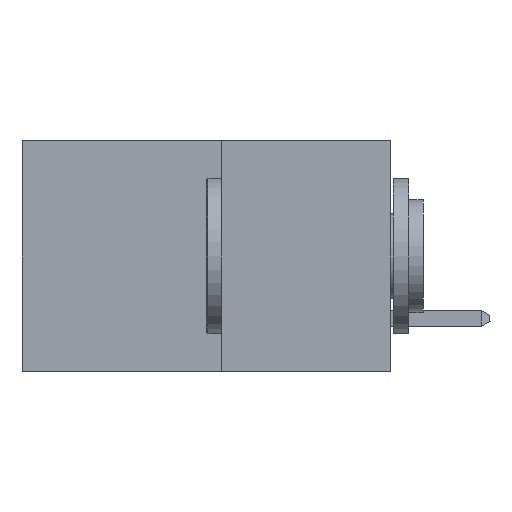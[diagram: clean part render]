
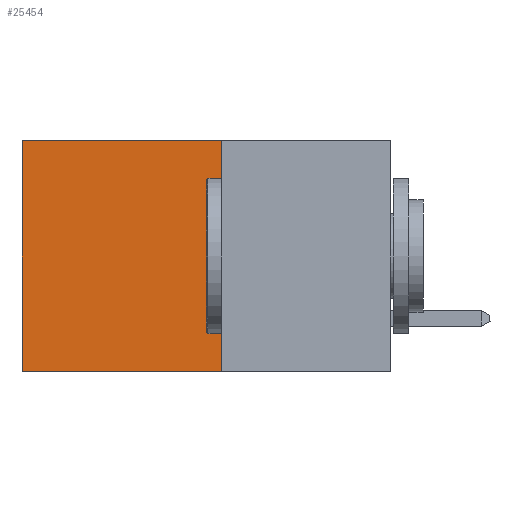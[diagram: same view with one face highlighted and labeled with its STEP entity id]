
A CAD part, left-side view. The second image highlights one B-rep face of the part: STEP entity #25454.
In plain terms, the highlighted planar face has unit normal (-1, 0, 0).
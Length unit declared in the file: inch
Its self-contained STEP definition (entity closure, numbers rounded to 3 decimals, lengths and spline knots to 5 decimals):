
#133 = EDGE_CURVE ( 'NONE', #9259, #26897, #26721, .T. ) ;
#818 = VECTOR ( 'NONE', #26434, 39.37008 ) ;
#1308 = AXIS2_PLACEMENT_3D ( 'NONE', #23926, #11339, #28965 ) ;
#1437 = ORIENTED_EDGE ( 'NONE', *, *, #10328, .F. ) ;
#1995 = ORIENTED_EDGE ( 'NONE', *, *, #133, .T. ) ;
#3621 = CARTESIAN_POINT ( 'NONE',  ( 0.277, 0.59, 0. ) ) ;
#3646 = ORIENTED_EDGE ( 'NONE', *, *, #11462, .F. ) ;
#4368 = EDGE_LOOP ( 'NONE', ( #1995, #3646, #1437, #27315 ) ) ;
#6079 = VERTEX_POINT ( 'NONE', #24299 ) ;
#6215 = PLANE ( 'NONE',  #1308 ) ;
#6647 = CARTESIAN_POINT ( 'NONE',  ( 0.277, 0.27, -0.37 ) ) ;
#6707 = VERTEX_POINT ( 'NONE', #6647 ) ;
#7480 = LINE ( 'NONE', #18878, #818 ) ;
#9259 = VERTEX_POINT ( 'NONE', #3621 ) ;
#10328 = EDGE_CURVE ( 'NONE', #6079, #6707, #25913, .T. ) ;
#11339 = DIRECTION ( 'NONE',  ( 1., 0., 0. ) ) ;
#11462 = EDGE_CURVE ( 'NONE', #6707, #26897, #15574, .T. ) ;
#12128 = DIRECTION ( 'NONE',  ( 0., 1., 0. ) ) ;
#12472 = CARTESIAN_POINT ( 'NONE',  ( 0.277, 0.59, -0.37 ) ) ;
#12903 = CARTESIAN_POINT ( 'NONE',  ( 0.277, 0.59, -0.37 ) ) ;
#13319 = VECTOR ( 'NONE', #15750, 39.37008 ) ;
#15390 = CARTESIAN_POINT ( 'NONE',  ( 0.277, 0.27, -0.37 ) ) ;
#15574 = LINE ( 'NONE', #22310, #28183 ) ;
#15750 = DIRECTION ( 'NONE',  ( 0., 0., -1. ) ) ;
#17946 = DIRECTION ( 'NONE',  ( 0., 0., -1. ) ) ;
#18878 = CARTESIAN_POINT ( 'NONE',  ( 0.277, 0.27, 0. ) ) ;
#22310 = CARTESIAN_POINT ( 'NONE',  ( 0.277, 0.27, -0.37 ) ) ;
#23926 = CARTESIAN_POINT ( 'NONE',  ( 0.277, 0.27, -0.37 ) ) ;
#24299 = CARTESIAN_POINT ( 'NONE',  ( 0.277, 0.27, 0. ) ) ;
#25454 = ADVANCED_FACE ( 'NONE', ( #32328 ), #6215, .F. ) ;
#25913 = LINE ( 'NONE', #15390, #30978 ) ;
#26434 = DIRECTION ( 'NONE',  ( 0., 1., 0. ) ) ;
#26721 = LINE ( 'NONE', #12903, #13319 ) ;
#26897 = VERTEX_POINT ( 'NONE', #12472 ) ;
#27277 = EDGE_CURVE ( 'NONE', #6079, #9259, #7480, .T. ) ;
#27315 = ORIENTED_EDGE ( 'NONE', *, *, #27277, .T. ) ;
#28183 = VECTOR ( 'NONE', #12128, 39.37008 ) ;
#28965 = DIRECTION ( 'NONE',  ( 0., 0., -1. ) ) ;
#30978 = VECTOR ( 'NONE', #17946, 39.37008 ) ;
#32328 = FACE_OUTER_BOUND ( 'NONE', #4368, .T. ) ;
